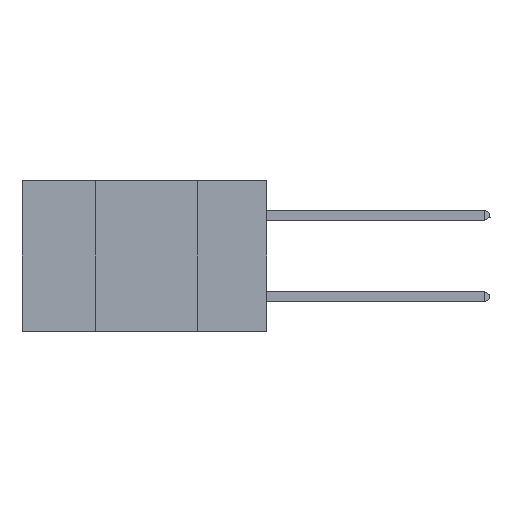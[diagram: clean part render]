
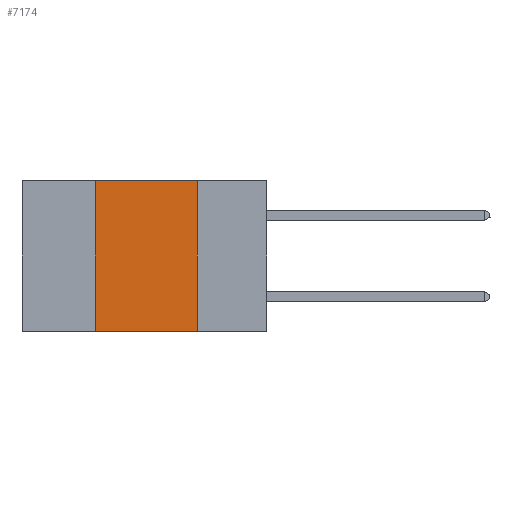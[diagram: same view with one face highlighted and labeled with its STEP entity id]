
A CAD part, left-side view. The second image highlights one B-rep face of the part: STEP entity #7174.
In plain terms, the highlighted planar face has unit normal (-1, 0, 0).
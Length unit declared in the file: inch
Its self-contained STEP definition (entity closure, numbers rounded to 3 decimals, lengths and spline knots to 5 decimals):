
#1943 = EDGE_CURVE ( 'NONE', #9997, #12407, #21033, .T. ) ;
#2104 = DIRECTION ( 'NONE',  ( 0., 0., -1. ) ) ;
#2646 = ORIENTED_EDGE ( 'NONE', *, *, #30798, .F. ) ;
#3673 = CARTESIAN_POINT ( 'NONE',  ( 0., 0.17, -0.37 ) ) ;
#4864 = VECTOR ( 'NONE', #24202, 39.37008 ) ;
#5448 = VECTOR ( 'NONE', #39550, 39.37008 ) ;
#6003 = CARTESIAN_POINT ( 'NONE',  ( 0., 0.42, -0.37 ) ) ;
#7174 = ADVANCED_FACE ( 'NONE', ( #14441 ), #30764, .F. ) ;
#7189 = LINE ( 'NONE', #7598, #31720 ) ;
#7598 = CARTESIAN_POINT ( 'NONE',  ( 0., 0.42, 0. ) ) ;
#9997 = VERTEX_POINT ( 'NONE', #35465 ) ;
#10277 = VECTOR ( 'NONE', #27099, 39.37008 ) ;
#12078 = EDGE_CURVE ( 'NONE', #25679, #9997, #37625, .T. ) ;
#12216 = ORIENTED_EDGE ( 'NONE', *, *, #1943, .F. ) ;
#12407 = VERTEX_POINT ( 'NONE', #3673 ) ;
#14441 = FACE_OUTER_BOUND ( 'NONE', #38866, .T. ) ;
#14981 = CARTESIAN_POINT ( 'NONE',  ( 0., 0.42, 0. ) ) ;
#16188 = EDGE_CURVE ( 'NONE', #35304, #12407, #20472, .T. ) ;
#17616 = DIRECTION ( 'NONE',  ( 0., 0., 1. ) ) ;
#20283 = AXIS2_PLACEMENT_3D ( 'NONE', #27622, #20927, #2104 ) ;
#20323 = ORIENTED_EDGE ( 'NONE', *, *, #12078, .F. ) ;
#20472 = LINE ( 'NONE', #23627, #5448 ) ;
#20927 = DIRECTION ( 'NONE',  ( 1., 0., 0. ) ) ;
#21033 = LINE ( 'NONE', #33397, #10277 ) ;
#21253 = ORIENTED_EDGE ( 'NONE', *, *, #16188, .T. ) ;
#23627 = CARTESIAN_POINT ( 'NONE',  ( 0., 0.6, -0.37 ) ) ;
#24202 = DIRECTION ( 'NONE',  ( 0., -1., 0. ) ) ;
#25679 = VERTEX_POINT ( 'NONE', #14981 ) ;
#27099 = DIRECTION ( 'NONE',  ( 0., 0., -1. ) ) ;
#27622 = CARTESIAN_POINT ( 'NONE',  ( 0., 0.6, 0. ) ) ;
#30764 = PLANE ( 'NONE',  #20283 ) ;
#30798 = EDGE_CURVE ( 'NONE', #35304, #25679, #7189, .T. ) ;
#31720 = VECTOR ( 'NONE', #17616, 39.37008 ) ;
#33397 = CARTESIAN_POINT ( 'NONE',  ( 0., 0.17, 0. ) ) ;
#34265 = CARTESIAN_POINT ( 'NONE',  ( 0., 0.6, 0. ) ) ;
#35304 = VERTEX_POINT ( 'NONE', #6003 ) ;
#35465 = CARTESIAN_POINT ( 'NONE',  ( 0., 0.17, 0. ) ) ;
#37625 = LINE ( 'NONE', #34265, #4864 ) ;
#38866 = EDGE_LOOP ( 'NONE', ( #12216, #20323, #2646, #21253 ) ) ;
#39550 = DIRECTION ( 'NONE',  ( 0., -1., 0. ) ) ;
